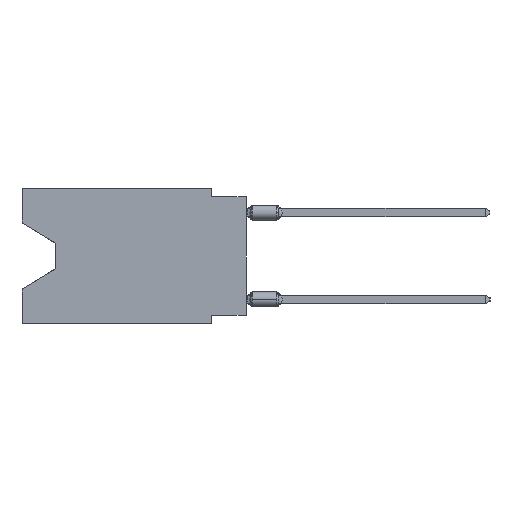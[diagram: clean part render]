
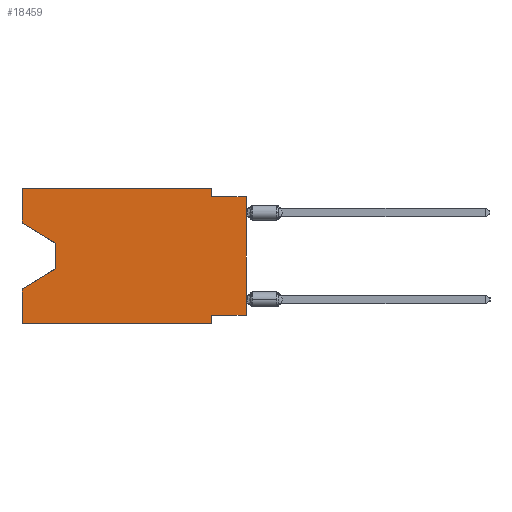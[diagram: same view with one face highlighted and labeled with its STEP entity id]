
A CAD part, left-side view. The second image highlights one B-rep face of the part: STEP entity #18459.
In plain terms, the highlighted planar face has unit normal (-1, 0, 0).
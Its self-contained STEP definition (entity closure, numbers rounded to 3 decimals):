
#1758 = ORIENTED_EDGE ( 'NONE', *, *, #18028, .T. ) ;
#2377 = ORIENTED_EDGE ( 'NONE', *, *, #26609, .F. ) ;
#2466 = VERTEX_POINT ( 'NONE', #21065 ) ;
#3049 = DIRECTION ( 'NONE',  ( 0., -1., 0. ) ) ;
#3168 = LINE ( 'NONE', #37162, #9743 ) ;
#3233 = CARTESIAN_POINT ( 'NONE',  ( 0., 0., 0. ) ) ;
#3421 = VERTEX_POINT ( 'NONE', #24215 ) ;
#3511 = DIRECTION ( 'NONE',  ( 0., -0.855, -0.519 ) ) ;
#3954 = ORIENTED_EDGE ( 'NONE', *, *, #11782, .T. ) ;
#4074 = CARTESIAN_POINT ( 'NONE',  ( 0., 16.383, -9.906 ) ) ;
#4767 = LINE ( 'NONE', #23967, #21177 ) ;
#4924 = ORIENTED_EDGE ( 'NONE', *, *, #15847, .F. ) ;
#5055 = EDGE_CURVE ( 'NONE', #33611, #30078, #16441, .T. ) ;
#5285 = ORIENTED_EDGE ( 'NONE', *, *, #19978, .F. ) ;
#5454 = VECTOR ( 'NONE', #35941, 1000. ) ;
#6221 = VERTEX_POINT ( 'NONE', #24436 ) ;
#7592 = DIRECTION ( 'NONE',  ( 0., 0., -1. ) ) ;
#9743 = VECTOR ( 'NONE', #18387, 1000. ) ;
#10769 = VECTOR ( 'NONE', #26178, 1000. ) ;
#11579 = AXIS2_PLACEMENT_3D ( 'NONE', #41838, #45092, #7592 ) ;
#11782 = EDGE_CURVE ( 'NONE', #27507, #2466, #13735, .T. ) ;
#12108 = CARTESIAN_POINT ( 'NONE',  ( 0., 0., -9.271 ) ) ;
#12226 = VERTEX_POINT ( 'NONE', #15102 ) ;
#13735 = LINE ( 'NONE', #3233, #23659 ) ;
#14602 = ORIENTED_EDGE ( 'NONE', *, *, #16681, .F. ) ;
#14671 = LINE ( 'NONE', #33421, #10769 ) ;
#14836 = PLANE ( 'NONE',  #11579 ) ;
#15102 = CARTESIAN_POINT ( 'NONE',  ( 0., 2.54, -9.906 ) ) ;
#15683 = CARTESIAN_POINT ( 'NONE',  ( 0., 16.383, -7.36 ) ) ;
#15755 = DIRECTION ( 'NONE',  ( 0., 0., -1. ) ) ;
#15847 = EDGE_CURVE ( 'NONE', #27507, #43295, #3168, .T. ) ;
#15928 = CARTESIAN_POINT ( 'NONE',  ( 0., 16.383, 0. ) ) ;
#16441 = LINE ( 'NONE', #32174, #5454 ) ;
#16681 = EDGE_CURVE ( 'NONE', #30078, #3421, #33966, .T. ) ;
#18028 = EDGE_CURVE ( 'NONE', #6221, #28766, #24175, .T. ) ;
#18387 = DIRECTION ( 'NONE',  ( 0., 1., 0. ) ) ;
#18459 = ADVANCED_FACE ( 'NONE', ( #26566 ), #14836, .F. ) ;
#18794 = VECTOR ( 'NONE', #3511, 1000. ) ;
#18828 = ORIENTED_EDGE ( 'NONE', *, *, #5055, .F. ) ;
#19480 = LINE ( 'NONE', #26502, #48379 ) ;
#19740 = LINE ( 'NONE', #42028, #29954 ) ;
#19978 = EDGE_CURVE ( 'NONE', #42006, #2466, #30508, .T. ) ;
#21065 = CARTESIAN_POINT ( 'NONE',  ( 0., 0., -0.635 ) ) ;
#21177 = VECTOR ( 'NONE', #15755, 1000. ) ;
#21753 = LINE ( 'NONE', #48533, #18794 ) ;
#22810 = CARTESIAN_POINT ( 'NONE',  ( 0., 13.97, -4.013 ) ) ;
#23659 = VECTOR ( 'NONE', #33472, 1000. ) ;
#23967 = CARTESIAN_POINT ( 'NONE',  ( 0., 13.97, -4.013 ) ) ;
#24175 = LINE ( 'NONE', #43216, #24279 ) ;
#24215 = CARTESIAN_POINT ( 'NONE',  ( 0., 2.54, 0. ) ) ;
#24279 = VECTOR ( 'NONE', #27033, 1000. ) ;
#24436 = CARTESIAN_POINT ( 'NONE',  ( 0., 13.97, -5.893 ) ) ;
#24869 = ORIENTED_EDGE ( 'NONE', *, *, #29642, .T. ) ;
#26178 = DIRECTION ( 'NONE',  ( 0., 0., -1. ) ) ;
#26227 = CARTESIAN_POINT ( 'NONE',  ( 0., 16.383, 0. ) ) ;
#26468 = DIRECTION ( 'NONE',  ( 0., -1., 0. ) ) ;
#26502 = CARTESIAN_POINT ( 'NONE',  ( 0., 16.383, -9.906 ) ) ;
#26566 = FACE_OUTER_BOUND ( 'NONE', #32348, .T. ) ;
#26609 = EDGE_CURVE ( 'NONE', #43295, #12226, #46065, .T. ) ;
#27033 = DIRECTION ( 'NONE',  ( 0., 0.855, -0.519 ) ) ;
#27507 = VERTEX_POINT ( 'NONE', #12108 ) ;
#28211 = EDGE_CURVE ( 'NONE', #33611, #40820, #21753, .T. ) ;
#28766 = VERTEX_POINT ( 'NONE', #15683 ) ;
#29590 = EDGE_CURVE ( 'NONE', #30473, #28766, #19740, .T. ) ;
#29642 = EDGE_CURVE ( 'NONE', #40820, #6221, #4767, .T. ) ;
#29954 = VECTOR ( 'NONE', #39000, 1000. ) ;
#30014 = CARTESIAN_POINT ( 'NONE',  ( 0., 0., -0.635 ) ) ;
#30078 = VERTEX_POINT ( 'NONE', #15928 ) ;
#30473 = VERTEX_POINT ( 'NONE', #4074 ) ;
#30508 = LINE ( 'NONE', #30014, #46792 ) ;
#31270 = CARTESIAN_POINT ( 'NONE',  ( 0., 2.54, -9.906 ) ) ;
#32174 = CARTESIAN_POINT ( 'NONE',  ( 0., 16.383, 0. ) ) ;
#32181 = VECTOR ( 'NONE', #26468, 1000. ) ;
#32348 = EDGE_LOOP ( 'NONE', ( #33936, #24869, #1758, #38930, #34112, #2377, #4924, #3954, #5285, #45567, #14602, #18828 ) ) ;
#33421 = CARTESIAN_POINT ( 'NONE',  ( 0., 2.54, 0. ) ) ;
#33472 = DIRECTION ( 'NONE',  ( 0., 0., 1. ) ) ;
#33611 = VERTEX_POINT ( 'NONE', #41481 ) ;
#33735 = CARTESIAN_POINT ( 'NONE',  ( 0., 2.54, -0.635 ) ) ;
#33936 = ORIENTED_EDGE ( 'NONE', *, *, #28211, .T. ) ;
#33966 = LINE ( 'NONE', #26227, #32181 ) ;
#34112 = ORIENTED_EDGE ( 'NONE', *, *, #45087, .T. ) ;
#34743 = DIRECTION ( 'NONE',  ( 0., -1., 0. ) ) ;
#35345 = EDGE_CURVE ( 'NONE', #3421, #42006, #14671, .T. ) ;
#35941 = DIRECTION ( 'NONE',  ( 0., 0., 1. ) ) ;
#37162 = CARTESIAN_POINT ( 'NONE',  ( 0., 0., -9.271 ) ) ;
#37870 = VECTOR ( 'NONE', #41824, 1000. ) ;
#38810 = CARTESIAN_POINT ( 'NONE',  ( 0., 2.54, -9.271 ) ) ;
#38930 = ORIENTED_EDGE ( 'NONE', *, *, #29590, .F. ) ;
#39000 = DIRECTION ( 'NONE',  ( 0., 0., 1. ) ) ;
#40820 = VERTEX_POINT ( 'NONE', #22810 ) ;
#41481 = CARTESIAN_POINT ( 'NONE',  ( 0., 16.383, -2.546 ) ) ;
#41824 = DIRECTION ( 'NONE',  ( 0., 0., -1. ) ) ;
#41838 = CARTESIAN_POINT ( 'NONE',  ( 0., 16.383, 0. ) ) ;
#42006 = VERTEX_POINT ( 'NONE', #33735 ) ;
#42028 = CARTESIAN_POINT ( 'NONE',  ( 0., 16.383, 0. ) ) ;
#43216 = CARTESIAN_POINT ( 'NONE',  ( 0., 13.97, -5.893 ) ) ;
#43295 = VERTEX_POINT ( 'NONE', #38810 ) ;
#45087 = EDGE_CURVE ( 'NONE', #30473, #12226, #19480, .T. ) ;
#45092 = DIRECTION ( 'NONE',  ( 1., 0., 0. ) ) ;
#45567 = ORIENTED_EDGE ( 'NONE', *, *, #35345, .F. ) ;
#46065 = LINE ( 'NONE', #31270, #37870 ) ;
#46792 = VECTOR ( 'NONE', #3049, 1000. ) ;
#48379 = VECTOR ( 'NONE', #34743, 1000. ) ;
#48533 = CARTESIAN_POINT ( 'NONE',  ( 0., 16.383, -2.546 ) ) ;
